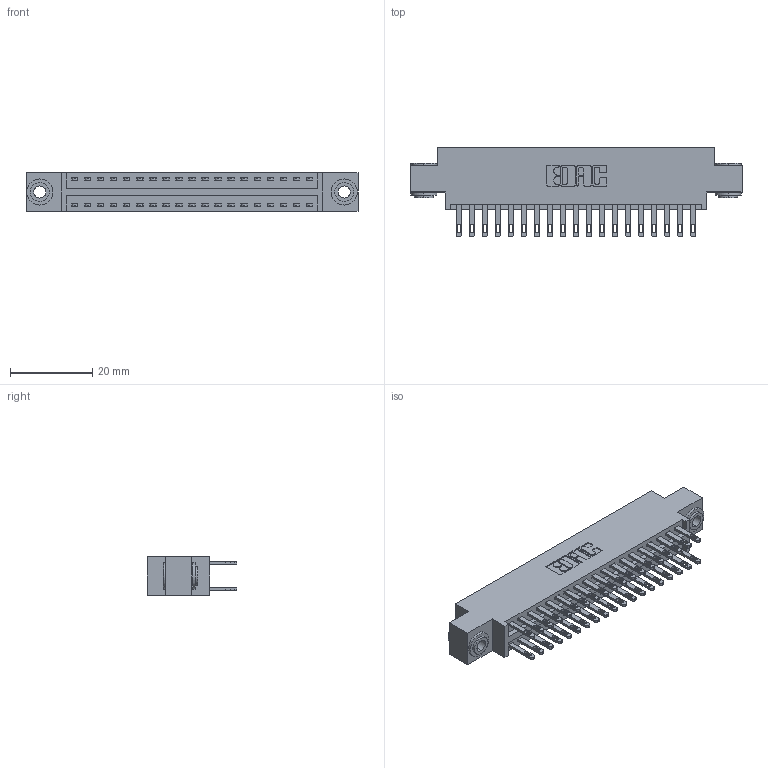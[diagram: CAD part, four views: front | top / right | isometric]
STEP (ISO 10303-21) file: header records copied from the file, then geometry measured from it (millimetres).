
FILE_DESCRIPTION (( 'STEP AP203' ), '1' );
FILE_NAME ('896-038-500-803.STEP', '2021-07-27T20:46:36', ( '' ), ( '' ), 'SwSTEP 2.0', 'SolidWorks 2020', '' );
FILE_SCHEMA (( 'CONFIG_CONTROL_DESIGN' ));
Length unit declared in the file: inch
Products named in the file (4): 846 Part_0.170 Offset - 0.156 Dia-TH; 345-250-002_345-250-002-102; 896-038-500-803; 345-292-001_345-293-100
Assembly tree (41 placements, depth 2):
  896-038-500-803
    846 Part_0.170 Offset - 0.156 Dia-TH
    345-292-001_345-293-100  x38
    345-250-002_345-250-002-102  x2
Bounding box: 80.9 x 21.84 x 9.4 mm (x, y, z)
Volume: 7690.9 mm3; surface area: 11001.7 mm2
Topology: 41 solids, 41 shells, 1988 faces, 6003 edges, 3998 vertices
Faces by surface type: plane 1192, cylinder 788, cone 8
Entity records: 16208 total; most frequent: CARTESIAN_POINT 2679, ORIENTED_EDGE 2606, DIRECTION 2445, EDGE_CURVE 1303, LINE 1067, VECTOR 1067, VERTEX_POINT 866, AXIS2_PLACEMENT_3D 689
